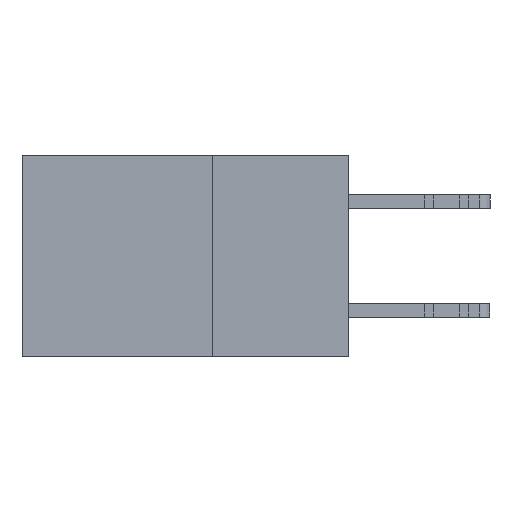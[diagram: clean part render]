
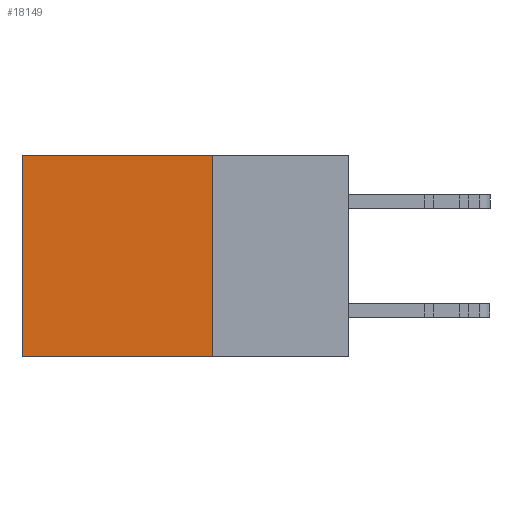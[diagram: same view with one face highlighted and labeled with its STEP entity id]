
A CAD part, left-side view. The second image highlights one B-rep face of the part: STEP entity #18149.
In plain terms, the highlighted planar face has unit normal (-1, 0, 0).
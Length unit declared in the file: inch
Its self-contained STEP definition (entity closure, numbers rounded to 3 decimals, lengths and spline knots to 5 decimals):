
#417 = FACE_OUTER_BOUND ( 'NONE', #10868, .T. ) ;
#836 = AXIS2_PLACEMENT_3D ( 'NONE', #12909, #10569, #27311 ) ;
#1549 = DIRECTION ( 'NONE',  ( 0., 1., 0. ) ) ;
#3133 = CARTESIAN_POINT ( 'NONE',  ( 0.298, 0.6, 0. ) ) ;
#3350 = DIRECTION ( 'NONE',  ( 0., 0., -1. ) ) ;
#4589 = CARTESIAN_POINT ( 'NONE',  ( 0.298, 0.6, -0.37 ) ) ;
#4884 = VERTEX_POINT ( 'NONE', #28224 ) ;
#7027 = ORIENTED_EDGE ( 'NONE', *, *, #21136, .F. ) ;
#7142 = EDGE_CURVE ( 'NONE', #15252, #21883, #17158, .T. ) ;
#7188 = CARTESIAN_POINT ( 'NONE',  ( 0.298, 0.25, -0.37 ) ) ;
#7574 = CARTESIAN_POINT ( 'NONE',  ( 0.298, 0.25, 0. ) ) ;
#7801 = VECTOR ( 'NONE', #1549, 39.37008 ) ;
#8347 = LINE ( 'NONE', #15466, #26009 ) ;
#8560 = LINE ( 'NONE', #11319, #7801 ) ;
#10569 = DIRECTION ( 'NONE',  ( 1., 0., 0. ) ) ;
#10652 = VECTOR ( 'NONE', #27186, 39.37008 ) ;
#10868 = EDGE_LOOP ( 'NONE', ( #17436, #7027, #28087, #15614 ) ) ;
#11319 = CARTESIAN_POINT ( 'NONE',  ( 0.298, 0.25, -0.37 ) ) ;
#12909 = CARTESIAN_POINT ( 'NONE',  ( 0.298, 0.25, 0. ) ) ;
#15252 = VERTEX_POINT ( 'NONE', #26348 ) ;
#15466 = CARTESIAN_POINT ( 'NONE',  ( 0.298, 0.25, 0. ) ) ;
#15614 = ORIENTED_EDGE ( 'NONE', *, *, #23434, .T. ) ;
#17158 = LINE ( 'NONE', #3133, #10652 ) ;
#17436 = ORIENTED_EDGE ( 'NONE', *, *, #7142, .T. ) ;
#18149 = ADVANCED_FACE ( 'NONE', ( #417 ), #22604, .F. ) ;
#21136 = EDGE_CURVE ( 'NONE', #30610, #21883, #8560, .T. ) ;
#21883 = VERTEX_POINT ( 'NONE', #4589 ) ;
#22005 = LINE ( 'NONE', #7574, #28277 ) ;
#22067 = DIRECTION ( 'NONE',  ( 0., 1., 0. ) ) ;
#22604 = PLANE ( 'NONE',  #836 ) ;
#23434 = EDGE_CURVE ( 'NONE', #4884, #15252, #22005, .T. ) ;
#24545 = EDGE_CURVE ( 'NONE', #4884, #30610, #8347, .T. ) ;
#26009 = VECTOR ( 'NONE', #3350, 39.37008 ) ;
#26348 = CARTESIAN_POINT ( 'NONE',  ( 0.298, 0.6, 0. ) ) ;
#27186 = DIRECTION ( 'NONE',  ( 0., 0., -1. ) ) ;
#27311 = DIRECTION ( 'NONE',  ( 0., 0., -1. ) ) ;
#28087 = ORIENTED_EDGE ( 'NONE', *, *, #24545, .F. ) ;
#28224 = CARTESIAN_POINT ( 'NONE',  ( 0.298, 0.25, 0. ) ) ;
#28277 = VECTOR ( 'NONE', #22067, 39.37008 ) ;
#30610 = VERTEX_POINT ( 'NONE', #7188 ) ;
